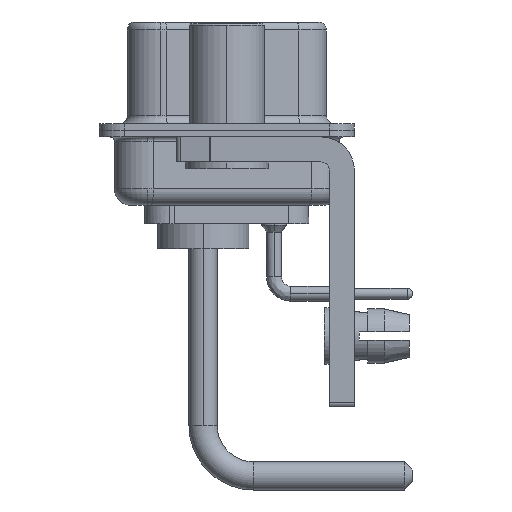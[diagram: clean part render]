
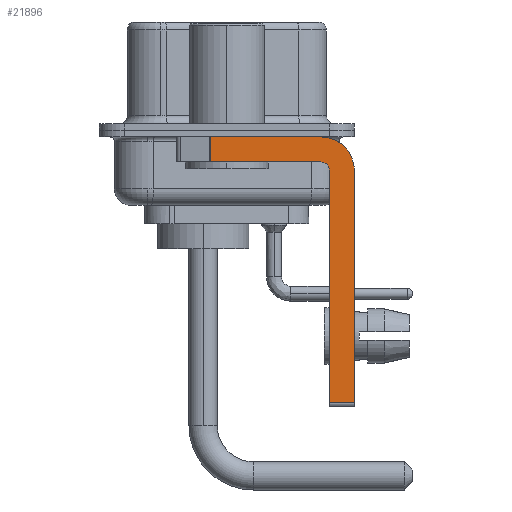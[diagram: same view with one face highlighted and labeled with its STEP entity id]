
A CAD part, left-side view. The second image highlights one B-rep face of the part: STEP entity #21896.
In plain terms, the highlighted planar face has unit normal (-1, 0, 0).
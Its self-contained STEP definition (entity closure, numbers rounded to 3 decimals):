
#165 = EDGE_CURVE ( 'NONE', #2115, #10975, #21523, .T. ) ;
#582 = DIRECTION ( 'NONE',  ( 0., 0., -1. ) ) ;
#729 = CARTESIAN_POINT ( 'NONE',  ( -2.9, -6.15, -16.6 ) ) ;
#1259 = CARTESIAN_POINT ( 'NONE',  ( -2.9, 3., -0.4 ) ) ;
#1896 = CARTESIAN_POINT ( 'NONE',  ( -2.9, -7.65, -2.4 ) ) ;
#2115 = VERTEX_POINT ( 'NONE', #21877 ) ;
#2255 = ORIENTED_EDGE ( 'NONE', *, *, #165, .F. ) ;
#2323 = PLANE ( 'NONE',  #18161 ) ;
#2359 = AXIS2_PLACEMENT_3D ( 'NONE', #4995, #26060, #8911 ) ;
#2427 = EDGE_CURVE ( 'NONE', #26374, #18092, #23650, .T. ) ;
#3178 = VECTOR ( 'NONE', #582, 1000. ) ;
#4040 = VECTOR ( 'NONE', #11431, 1000. ) ;
#4995 = CARTESIAN_POINT ( 'NONE',  ( -2.9, -5.65, -2.4 ) ) ;
#6231 = CARTESIAN_POINT ( 'NONE',  ( -2.9, -6.15, -2.4 ) ) ;
#6260 = EDGE_CURVE ( 'NONE', #11167, #13035, #7132, .T. ) ;
#6370 = DIRECTION ( 'NONE',  ( 1., 0., 0. ) ) ;
#7132 = LINE ( 'NONE', #18077, #4040 ) ;
#7465 = CARTESIAN_POINT ( 'NONE',  ( -2.9, -7.65, -2.4 ) ) ;
#7612 = EDGE_CURVE ( 'NONE', #18816, #18092, #9230, .T. ) ;
#8891 = VECTOR ( 'NONE', #13850, 1000. ) ;
#8911 = DIRECTION ( 'NONE',  ( 0., 0., 1. ) ) ;
#9230 = LINE ( 'NONE', #15487, #3178 ) ;
#9264 = ORIENTED_EDGE ( 'NONE', *, *, #24084, .F. ) ;
#9286 = CARTESIAN_POINT ( 'NONE',  ( -2.9, -7.65, -16.35 ) ) ;
#9491 = LINE ( 'NONE', #1259, #24362 ) ;
#10685 = CARTESIAN_POINT ( 'NONE',  ( -2.9, -5.65, -2.4 ) ) ;
#10924 = CARTESIAN_POINT ( 'NONE',  ( -2.9, -5.65, -1.9 ) ) ;
#10975 = VERTEX_POINT ( 'NONE', #1896 ) ;
#11098 = EDGE_CURVE ( 'NONE', #12903, #26374, #23644, .T. ) ;
#11167 = VERTEX_POINT ( 'NONE', #17904 ) ;
#11431 = DIRECTION ( 'NONE',  ( 0., -1., 0. ) ) ;
#11454 = VECTOR ( 'NONE', #17422, 1000. ) ;
#11776 = CARTESIAN_POINT ( 'NONE',  ( -2.9, -5.65, -2.4 ) ) ;
#12108 = DIRECTION ( 'NONE',  ( 0., -1., 0. ) ) ;
#12269 = CARTESIAN_POINT ( 'NONE',  ( -2.9, -5.65, -1.9 ) ) ;
#12845 = LINE ( 'NONE', #729, #11454 ) ;
#12903 = VERTEX_POINT ( 'NONE', #6231 ) ;
#13035 = VERTEX_POINT ( 'NONE', #9286 ) ;
#13850 = DIRECTION ( 'NONE',  ( 0., 0., -1. ) ) ;
#14749 = ORIENTED_EDGE ( 'NONE', *, *, #7612, .T. ) ;
#15144 = FACE_OUTER_BOUND ( 'NONE', #25740, .T. ) ;
#15487 = CARTESIAN_POINT ( 'NONE',  ( -2.9, 0.978, -1.9 ) ) ;
#16289 = VECTOR ( 'NONE', #18965, 1000. ) ;
#17093 = AXIS2_PLACEMENT_3D ( 'NONE', #11776, #24241, #19976 ) ;
#17422 = DIRECTION ( 'NONE',  ( 0., 0., 1. ) ) ;
#17904 = CARTESIAN_POINT ( 'NONE',  ( -2.9, -6.15, -16.35 ) ) ;
#18077 = CARTESIAN_POINT ( 'NONE',  ( -2.9, -5.65, -16.35 ) ) ;
#18092 = VERTEX_POINT ( 'NONE', #19145 ) ;
#18123 = ORIENTED_EDGE ( 'NONE', *, *, #6260, .T. ) ;
#18161 = AXIS2_PLACEMENT_3D ( 'NONE', #10685, #6370, #25352 ) ;
#18692 = EDGE_CURVE ( 'NONE', #11167, #12903, #12845, .T. ) ;
#18816 = VERTEX_POINT ( 'NONE', #19375 ) ;
#18965 = DIRECTION ( 'NONE',  ( 0., 1., 0. ) ) ;
#19145 = CARTESIAN_POINT ( 'NONE',  ( -2.9, 0.978, -1.9 ) ) ;
#19375 = CARTESIAN_POINT ( 'NONE',  ( -2.9, 0.978, -0.4 ) ) ;
#19976 = DIRECTION ( 'NONE',  ( 0., 0., -1. ) ) ;
#20136 = ORIENTED_EDGE ( 'NONE', *, *, #18692, .F. ) ;
#20507 = ORIENTED_EDGE ( 'NONE', *, *, #2427, .F. ) ;
#20630 = LINE ( 'NONE', #7465, #8891 ) ;
#21523 = CIRCLE ( 'NONE', #17093, 2. ) ;
#21877 = CARTESIAN_POINT ( 'NONE',  ( -2.9, -5.65, -0.4 ) ) ;
#21896 = ADVANCED_FACE ( 'NONE', ( #15144 ), #2323, .F. ) ;
#21930 = ORIENTED_EDGE ( 'NONE', *, *, #11098, .F. ) ;
#22292 = EDGE_CURVE ( 'NONE', #10975, #13035, #20630, .T. ) ;
#23644 = CIRCLE ( 'NONE', #2359, 0.5 ) ;
#23650 = LINE ( 'NONE', #10924, #16289 ) ;
#24084 = EDGE_CURVE ( 'NONE', #18816, #2115, #9491, .T. ) ;
#24241 = DIRECTION ( 'NONE',  ( 1., 0., 0. ) ) ;
#24362 = VECTOR ( 'NONE', #12108, 1000. ) ;
#25352 = DIRECTION ( 'NONE',  ( 0., 0., -1. ) ) ;
#25740 = EDGE_LOOP ( 'NONE', ( #9264, #14749, #20507, #21930, #20136, #18123, #27317, #2255 ) ) ;
#26060 = DIRECTION ( 'NONE',  ( -1., 0., 0. ) ) ;
#26374 = VERTEX_POINT ( 'NONE', #12269 ) ;
#27317 = ORIENTED_EDGE ( 'NONE', *, *, #22292, .F. ) ;
